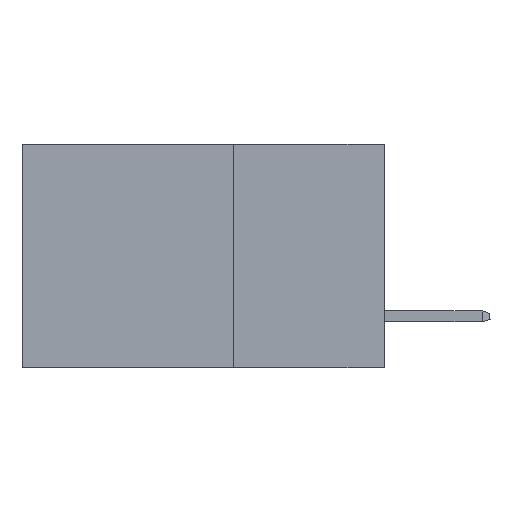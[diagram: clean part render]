
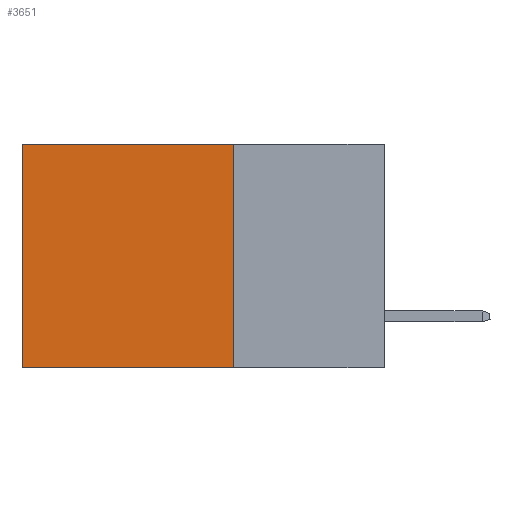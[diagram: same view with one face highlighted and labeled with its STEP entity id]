
A CAD part, left-side view. The second image highlights one B-rep face of the part: STEP entity #3651.
In plain terms, the highlighted planar face has unit normal (-1, 0, 0).
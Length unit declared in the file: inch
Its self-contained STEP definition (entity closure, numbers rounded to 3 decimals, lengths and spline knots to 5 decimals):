
#14 = DIRECTION ( 'NONE',  ( 0., 0., -1. ) ) ;
#553 = CARTESIAN_POINT ( 'NONE',  ( 0.2615, 0.25, -0.37 ) ) ;
#675 = ORIENTED_EDGE ( 'NONE', *, *, #707, .F. ) ;
#707 = EDGE_CURVE ( 'NONE', #6599, #1331, #1459, .T. ) ;
#939 = EDGE_CURVE ( 'NONE', #6599, #14223, #14248, .T. ) ;
#1331 = VERTEX_POINT ( 'NONE', #553 ) ;
#1393 = VECTOR ( 'NONE', #10737, 39.37008 ) ;
#1459 = LINE ( 'NONE', #2285, #5500 ) ;
#2016 = EDGE_CURVE ( 'NONE', #1331, #5847, #9770, .T. ) ;
#2266 = CARTESIAN_POINT ( 'NONE',  ( 0.2615, 0.25, 0. ) ) ;
#2285 = CARTESIAN_POINT ( 'NONE',  ( 0.2615, 0.25, -0.37 ) ) ;
#2509 = PLANE ( 'NONE',  #3450 ) ;
#2713 = CARTESIAN_POINT ( 'NONE',  ( 0.2615, 0.25, 0. ) ) ;
#3253 = ORIENTED_EDGE ( 'NONE', *, *, #2016, .F. ) ;
#3450 = AXIS2_PLACEMENT_3D ( 'NONE', #15372, #4850, #14 ) ;
#3651 = ADVANCED_FACE ( 'NONE', ( #9191 ), #2509, .F. ) ;
#3684 = CARTESIAN_POINT ( 'NONE',  ( 0.2615, 0.6, -0.37 ) ) ;
#4512 = EDGE_LOOP ( 'NONE', ( #4844, #3253, #675, #12628 ) ) ;
#4844 = ORIENTED_EDGE ( 'NONE', *, *, #6919, .T. ) ;
#4850 = DIRECTION ( 'NONE',  ( 1., 0., 0. ) ) ;
#5500 = VECTOR ( 'NONE', #10368, 39.37008 ) ;
#5675 = DIRECTION ( 'NONE',  ( 0., 1., 0. ) ) ;
#5847 = VERTEX_POINT ( 'NONE', #8065 ) ;
#6490 = CARTESIAN_POINT ( 'NONE',  ( 0.2615, 0.25, -0.37 ) ) ;
#6599 = VERTEX_POINT ( 'NONE', #2713 ) ;
#6734 = VECTOR ( 'NONE', #14796, 39.37008 ) ;
#6919 = EDGE_CURVE ( 'NONE', #14223, #5847, #12895, .T. ) ;
#8065 = CARTESIAN_POINT ( 'NONE',  ( 0.2615, 0.6, -0.37 ) ) ;
#9191 = FACE_OUTER_BOUND ( 'NONE', #4512, .T. ) ;
#9770 = LINE ( 'NONE', #6490, #6734 ) ;
#10368 = DIRECTION ( 'NONE',  ( 0., 0., -1. ) ) ;
#10737 = DIRECTION ( 'NONE',  ( 0., 0., -1. ) ) ;
#11092 = VECTOR ( 'NONE', #5675, 39.37008 ) ;
#12628 = ORIENTED_EDGE ( 'NONE', *, *, #939, .T. ) ;
#12895 = LINE ( 'NONE', #3684, #1393 ) ;
#14223 = VERTEX_POINT ( 'NONE', #14297 ) ;
#14248 = LINE ( 'NONE', #2266, #11092 ) ;
#14297 = CARTESIAN_POINT ( 'NONE',  ( 0.2615, 0.6, 0. ) ) ;
#14796 = DIRECTION ( 'NONE',  ( 0., 1., 0. ) ) ;
#15372 = CARTESIAN_POINT ( 'NONE',  ( 0.2615, 0.25, -0.37 ) ) ;
